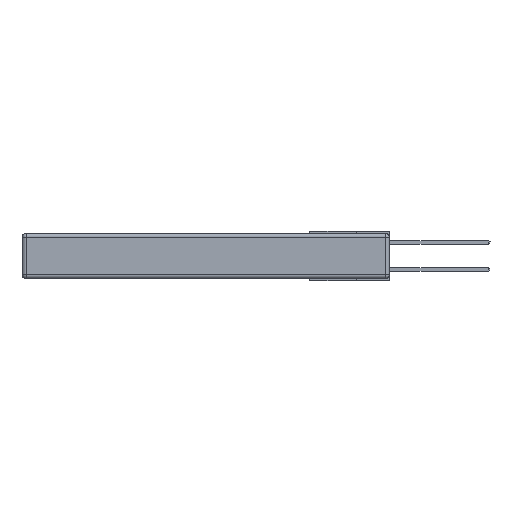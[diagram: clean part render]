
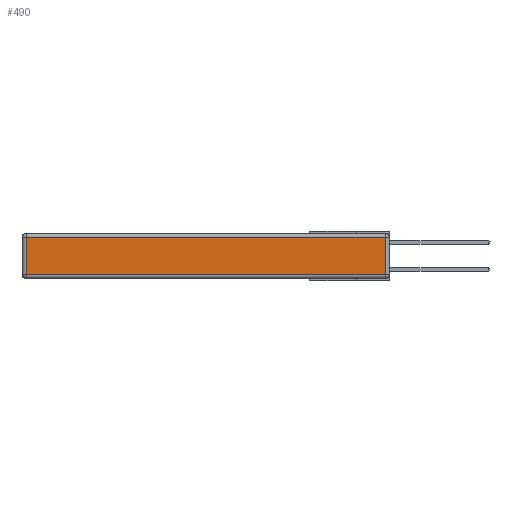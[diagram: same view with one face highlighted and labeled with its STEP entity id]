
A CAD part, left-side view. The second image highlights one B-rep face of the part: STEP entity #490.
In plain terms, the highlighted planar face has unit normal (-1, 0, 0).
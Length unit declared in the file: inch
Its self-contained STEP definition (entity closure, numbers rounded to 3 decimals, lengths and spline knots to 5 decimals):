
#5 = CARTESIAN_POINT ( 'NONE',  ( 0., 2.75, -0.03 ) ) ;
#407 = DIRECTION ( 'NONE',  ( 0., 0., 1. ) ) ;
#435 = ORIENTED_EDGE ( 'NONE', *, *, #5585, .T. ) ;
#490 = ADVANCED_FACE ( 'NONE', ( #14577 ), #9492, .T. ) ;
#1716 = VERTEX_POINT ( 'NONE', #5075 ) ;
#3677 = ORIENTED_EDGE ( 'NONE', *, *, #13722, .T. ) ;
#3918 = EDGE_CURVE ( 'NONE', #4871, #1716, #16630, .T. ) ;
#4871 = VERTEX_POINT ( 'NONE', #9442 ) ;
#5075 = CARTESIAN_POINT ( 'NONE',  ( 0., 0.03, -0.313 ) ) ;
#5392 = DIRECTION ( 'NONE',  ( -1., 0., 0. ) ) ;
#5585 = EDGE_CURVE ( 'NONE', #10737, #15415, #11673, .T. ) ;
#6282 = DIRECTION ( 'NONE',  ( 0., -1., 0. ) ) ;
#6454 = LINE ( 'NONE', #20115, #9236 ) ;
#6639 = EDGE_CURVE ( 'NONE', #15415, #4871, #20914, .T. ) ;
#6651 = DIRECTION ( 'NONE',  ( 0., 0., -1. ) ) ;
#7860 = ORIENTED_EDGE ( 'NONE', *, *, #6639, .T. ) ;
#8079 = DIRECTION ( 'NONE',  ( 0., 1., 0. ) ) ;
#8291 = CARTESIAN_POINT ( 'NONE',  ( 0., 2.72, -0.343 ) ) ;
#8386 = EDGE_LOOP ( 'NONE', ( #12843, #3677, #435, #7860 ) ) ;
#8676 = VECTOR ( 'NONE', #8079, 39.37008 ) ;
#9236 = VECTOR ( 'NONE', #13646, 39.37008 ) ;
#9442 = CARTESIAN_POINT ( 'NONE',  ( 0., 2.72, -0.313 ) ) ;
#9492 = PLANE ( 'NONE',  #19243 ) ;
#10737 = VERTEX_POINT ( 'NONE', #15725 ) ;
#11191 = CARTESIAN_POINT ( 'NONE',  ( 0., 0., -0.343 ) ) ;
#11673 = LINE ( 'NONE', #5, #8676 ) ;
#12840 = CARTESIAN_POINT ( 'NONE',  ( 0., 0., -0.313 ) ) ;
#12843 = ORIENTED_EDGE ( 'NONE', *, *, #3918, .T. ) ;
#13646 = DIRECTION ( 'NONE',  ( 0., 0., 1. ) ) ;
#13722 = EDGE_CURVE ( 'NONE', #1716, #10737, #6454, .T. ) ;
#14577 = FACE_OUTER_BOUND ( 'NONE', #8386, .T. ) ;
#14720 = VECTOR ( 'NONE', #6651, 39.37008 ) ;
#15205 = CARTESIAN_POINT ( 'NONE',  ( 0., 2.72, -0.03 ) ) ;
#15415 = VERTEX_POINT ( 'NONE', #15205 ) ;
#15725 = CARTESIAN_POINT ( 'NONE',  ( 0., 0.03, -0.03 ) ) ;
#16630 = LINE ( 'NONE', #12840, #20774 ) ;
#19243 = AXIS2_PLACEMENT_3D ( 'NONE', #11191, #5392, #407 ) ;
#20115 = CARTESIAN_POINT ( 'NONE',  ( 0., 0.03, -0.343 ) ) ;
#20774 = VECTOR ( 'NONE', #6282, 39.37008 ) ;
#20914 = LINE ( 'NONE', #8291, #14720 ) ;
